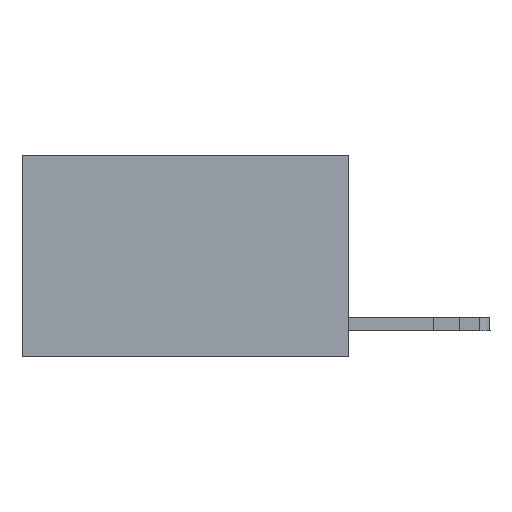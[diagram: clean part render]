
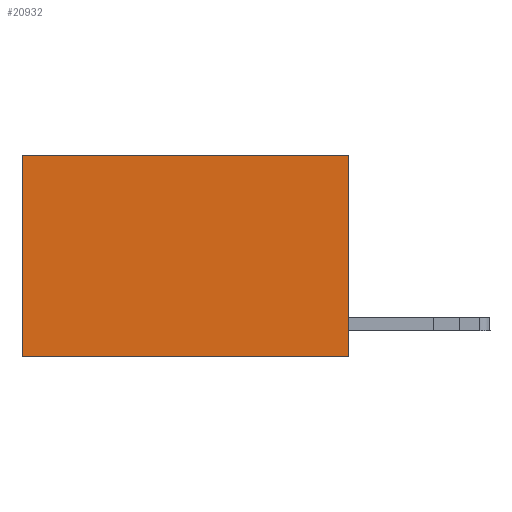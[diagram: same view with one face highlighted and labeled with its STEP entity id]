
A CAD part, left-side view. The second image highlights one B-rep face of the part: STEP entity #20932.
In plain terms, the highlighted planar face has unit normal (-1, 0, 0).
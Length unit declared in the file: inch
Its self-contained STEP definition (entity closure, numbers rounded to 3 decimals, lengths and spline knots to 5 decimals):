
#1089 = EDGE_LOOP ( 'NONE', ( #3763, #14445, #5738, #12684 ) ) ;
#1867 = VERTEX_POINT ( 'NONE', #7995 ) ;
#1915 = DIRECTION ( 'NONE',  ( 0., 0., -1. ) ) ;
#2468 = DIRECTION ( 'NONE',  ( 0., 1., 0. ) ) ;
#3763 = ORIENTED_EDGE ( 'NONE', *, *, #21150, .T. ) ;
#3999 = CARTESIAN_POINT ( 'NONE',  ( 0.2625, 0., -0.37 ) ) ;
#4376 = EDGE_CURVE ( 'NONE', #18881, #18800, #6115, .T. ) ;
#4689 = CARTESIAN_POINT ( 'NONE',  ( 0.2625, 0., 0. ) ) ;
#5738 = ORIENTED_EDGE ( 'NONE', *, *, #14176, .F. ) ;
#6115 = LINE ( 'NONE', #7904, #16665 ) ;
#6352 = CARTESIAN_POINT ( 'NONE',  ( 0.2625, 0., 0. ) ) ;
#6526 = CARTESIAN_POINT ( 'NONE',  ( 0.2625, 0.6, 0. ) ) ;
#7807 = PLANE ( 'NONE',  #14409 ) ;
#7904 = CARTESIAN_POINT ( 'NONE',  ( 0.2625, 0., -0.37 ) ) ;
#7995 = CARTESIAN_POINT ( 'NONE',  ( 0.2625, 0., 0. ) ) ;
#8681 = LINE ( 'NONE', #12208, #12677 ) ;
#9972 = VERTEX_POINT ( 'NONE', #6526 ) ;
#10232 = DIRECTION ( 'NONE',  ( 0., 0., -1. ) ) ;
#11204 = VECTOR ( 'NONE', #2468, 39.37008 ) ;
#12208 = CARTESIAN_POINT ( 'NONE',  ( 0.2625, 0.6, 0. ) ) ;
#12677 = VECTOR ( 'NONE', #1915, 39.37008 ) ;
#12684 = ORIENTED_EDGE ( 'NONE', *, *, #19820, .T. ) ;
#13078 = FACE_OUTER_BOUND ( 'NONE', #1089, .T. ) ;
#14176 = EDGE_CURVE ( 'NONE', #1867, #18881, #18747, .T. ) ;
#14409 = AXIS2_PLACEMENT_3D ( 'NONE', #4689, #14508, #14746 ) ;
#14445 = ORIENTED_EDGE ( 'NONE', *, *, #4376, .F. ) ;
#14508 = DIRECTION ( 'NONE',  ( 1., 0., 0. ) ) ;
#14746 = DIRECTION ( 'NONE',  ( 0., 0., -1. ) ) ;
#16665 = VECTOR ( 'NONE', #21354, 39.37008 ) ;
#17387 = VECTOR ( 'NONE', #10232, 39.37008 ) ;
#18747 = LINE ( 'NONE', #20605, #17387 ) ;
#18800 = VERTEX_POINT ( 'NONE', #20973 ) ;
#18881 = VERTEX_POINT ( 'NONE', #3999 ) ;
#19820 = EDGE_CURVE ( 'NONE', #1867, #9972, #21475, .T. ) ;
#20605 = CARTESIAN_POINT ( 'NONE',  ( 0.2625, 0., 0. ) ) ;
#20932 = ADVANCED_FACE ( 'NONE', ( #13078 ), #7807, .F. ) ;
#20973 = CARTESIAN_POINT ( 'NONE',  ( 0.2625, 0.6, -0.37 ) ) ;
#21150 = EDGE_CURVE ( 'NONE', #9972, #18800, #8681, .T. ) ;
#21354 = DIRECTION ( 'NONE',  ( 0., 1., 0. ) ) ;
#21475 = LINE ( 'NONE', #6352, #11204 ) ;
